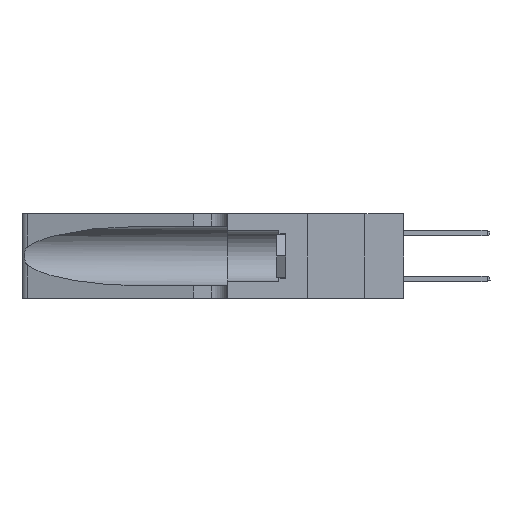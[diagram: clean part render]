
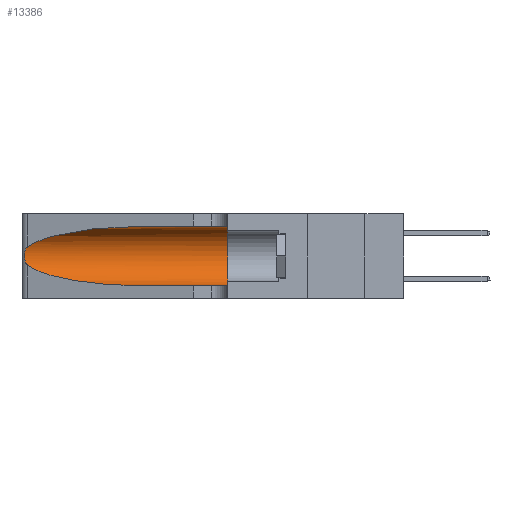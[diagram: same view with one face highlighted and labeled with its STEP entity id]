
A CAD part, left-side view. The second image highlights one B-rep face of the part: STEP entity #13386.
In plain terms, the highlighted cylindrical face has radius 3.308 mm (diameter 6.617 mm), a partial arc.
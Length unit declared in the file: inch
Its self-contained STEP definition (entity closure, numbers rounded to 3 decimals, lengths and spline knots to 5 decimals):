
#2082 = VERTEX_POINT ( 'NONE', #26902 ) ;
#2106 = EDGE_CURVE ( 'NONE', #43480, #2082, #8364, .T. ) ;
#2282 = AXIS2_PLACEMENT_3D ( 'NONE', #31212, #20043, #46346 ) ;
#2518 = CARTESIAN_POINT ( 'NONE',  ( 0.25639, 1.23184, 0.21858 ) ) ;
#4357 = CARTESIAN_POINT ( 'NONE',  ( 0.2373, 1.15595, 0.28018 ) ) ;
#4795 = DIRECTION ( 'NONE',  ( 0., -1., 0. ) ) ;
#5530 = CARTESIAN_POINT ( 'NONE',  ( 0.1305, 0.72297, 0.05475 ) ) ;
#5622 = VERTEX_POINT ( 'NONE', #33746 ) ;
#6374 = CARTESIAN_POINT ( 'NONE',  ( 0.25854, 1.2359, 0.20912 ) ) ;
#6934 = B_SPLINE_CURVE_WITH_KNOTS ( 'NONE', 3,
 ( #44008, #32668, #2518, #29024, #6374, #32831, #10190, #36622, #14015, #40368, #17830, #44166, #21634, #47950 ),
 .UNSPECIFIED., .F., .F.,
 ( 4, 2, 2, 2, 2, 2, 4 ),
 ( 0., 0.00027, 0.00053, 0.00107, 0.0016, 0.00187, 0.00214 ),
 .UNSPECIFIED. ) ;
#8364 = LINE ( 'NONE', #42034, #17282 ) ;
#10148 = CIRCLE ( 'NONE', #28569, 0.13025 ) ;
#10190 = CARTESIAN_POINT ( 'NONE',  ( 0.26075, 1.23896, 0.19203 ) ) ;
#13386 = ADVANCED_FACE ( 'NONE', ( #47611 ), #27585, .F. ) ;
#14015 = CARTESIAN_POINT ( 'NONE',  ( 0.26017, 1.23833, 0.17102 ) ) ;
#14213 = VECTOR ( 'NONE', #4795, 39.37008 ) ;
#15354 = CARTESIAN_POINT ( 'NONE',  ( 0.25487, 1.22718, 0.14631 ) ) ;
#15713 = CARTESIAN_POINT ( 'NONE',  ( 0.1305, 0.72297, 0.31525 ) ) ;
#15753 =( BOUNDED_CURVE ( )  B_SPLINE_CURVE ( 3, ( #20656, #20484, #28211, #5530 ),
 .UNSPECIFIED., .F., .F. ) 
 B_SPLINE_CURVE_WITH_KNOTS ( ( 4, 4 ),
 ( 3.44316, 4.71239 ),
 .UNSPECIFIED. ) 
 CURVE ( )  GEOMETRIC_REPRESENTATION_ITEM ( )  RATIONAL_B_SPLINE_CURVE ( ( 1., 0.87, 0.87, 1. ) ) 
 REPRESENTATION_ITEM ( '' )  );
#16607 = ORIENTED_EDGE ( 'NONE', *, *, #43605, .T. ) ;
#17282 = VECTOR ( 'NONE', #27069, 39.37008 ) ;
#17830 = CARTESIAN_POINT ( 'NONE',  ( 0.25789, 1.23486, 0.15765 ) ) ;
#19505 = CARTESIAN_POINT ( 'NONE',  ( 0.18966, 0.96281, 0.31525 ) ) ;
#19989 = CARTESIAN_POINT ( 'NONE',  ( 0.1305, 0.72297, 0.05475 ) ) ;
#20043 = DIRECTION ( 'NONE',  ( 0., -1., 0. ) ) ;
#20484 = CARTESIAN_POINT ( 'NONE',  ( 0.2373, 1.15595, 0.08982 ) ) ;
#20656 = CARTESIAN_POINT ( 'NONE',  ( 0.25487, 1.22718, 0.14631 ) ) ;
#20805 = DIRECTION ( 'NONE',  ( 0., 1., 0. ) ) ;
#21634 = CARTESIAN_POINT ( 'NONE',  ( 0.25555, 1.22993, 0.14849 ) ) ;
#24265 = CARTESIAN_POINT ( 'NONE',  ( 0.1305, 0.35, 0.31525 ) ) ;
#25650 = EDGE_CURVE ( 'NONE', #5622, #43592, #40740, .T. ) ;
#26902 = CARTESIAN_POINT ( 'NONE',  ( 0.1305, 0.35, 0.05475 ) ) ;
#27069 = DIRECTION ( 'NONE',  ( 0., -1., 0. ) ) ;
#27497 = CARTESIAN_POINT ( 'NONE',  ( 0.1305, 1.61858, 0.31525 ) ) ;
#27585 = CYLINDRICAL_SURFACE ( 'NONE', #2282, 0.13025 ) ;
#28211 = CARTESIAN_POINT ( 'NONE',  ( 0.18966, 0.96281, 0.05475 ) ) ;
#28569 = AXIS2_PLACEMENT_3D ( 'NONE', #43335, #20805, #47102 ) ;
#29024 = CARTESIAN_POINT ( 'NONE',  ( 0.25787, 1.23484, 0.2124 ) ) ;
#29061 = EDGE_CURVE ( 'NONE', #5622, #45926, #33306, .T. ) ;
#30831 = CARTESIAN_POINT ( 'NONE',  ( 0.25487, 1.22718, 0.22369 ) ) ;
#31212 = CARTESIAN_POINT ( 'NONE',  ( 0.1305, 1.61858, 0.185 ) ) ;
#32668 = CARTESIAN_POINT ( 'NONE',  ( 0.25555, 1.22994, 0.2215 ) ) ;
#32831 = CARTESIAN_POINT ( 'NONE',  ( 0.26018, 1.23835, 0.19895 ) ) ;
#33127 = ORIENTED_EDGE ( 'NONE', *, *, #29061, .T. ) ;
#33306 =( BOUNDED_CURVE ( )  B_SPLINE_CURVE ( 3, ( #15713, #19505, #4357, #30831 ),
 .UNSPECIFIED., .F., .T. ) 
 B_SPLINE_CURVE_WITH_KNOTS ( ( 4, 4 ),
 ( 1.5708, 2.84003 ),
 .UNSPECIFIED. ) 
 CURVE ( )  GEOMETRIC_REPRESENTATION_ITEM ( )  RATIONAL_B_SPLINE_CURVE ( ( 1., 0.87, 0.87, 1. ) ) 
 REPRESENTATION_ITEM ( '' )  );
#33746 = CARTESIAN_POINT ( 'NONE',  ( 0.1305, 0.72297, 0.31525 ) ) ;
#34301 = ORIENTED_EDGE ( 'NONE', *, *, #43754, .T. ) ;
#36622 = CARTESIAN_POINT ( 'NONE',  ( 0.26075, 1.23896, 0.178 ) ) ;
#39078 = EDGE_LOOP ( 'NONE', ( #33127, #34301, #16607, #46632, #47844, #40175 ) ) ;
#40175 = ORIENTED_EDGE ( 'NONE', *, *, #25650, .F. ) ;
#40368 = CARTESIAN_POINT ( 'NONE',  ( 0.25856, 1.23593, 0.16098 ) ) ;
#40740 = LINE ( 'NONE', #27497, #14213 ) ;
#41100 = EDGE_CURVE ( 'NONE', #43592, #2082, #10148, .T. ) ;
#42034 = CARTESIAN_POINT ( 'NONE',  ( 0.1305, 1.61858, 0.05475 ) ) ;
#43335 = CARTESIAN_POINT ( 'NONE',  ( 0.1305, 0.35, 0.185 ) ) ;
#43480 = VERTEX_POINT ( 'NONE', #19989 ) ;
#43592 = VERTEX_POINT ( 'NONE', #24265 ) ;
#43605 = EDGE_CURVE ( 'NONE', #45218, #43480, #15753, .T. ) ;
#43752 = CARTESIAN_POINT ( 'NONE',  ( 0.25487, 1.22718, 0.22369 ) ) ;
#43754 = EDGE_CURVE ( 'NONE', #45926, #45218, #6934, .T. ) ;
#44008 = CARTESIAN_POINT ( 'NONE',  ( 0.25487, 1.22718, 0.22369 ) ) ;
#44166 = CARTESIAN_POINT ( 'NONE',  ( 0.25639, 1.23186, 0.15144 ) ) ;
#45218 = VERTEX_POINT ( 'NONE', #15354 ) ;
#45926 = VERTEX_POINT ( 'NONE', #43752 ) ;
#46346 = DIRECTION ( 'NONE',  ( 0., 0., -1. ) ) ;
#46632 = ORIENTED_EDGE ( 'NONE', *, *, #2106, .T. ) ;
#47102 = DIRECTION ( 'NONE',  ( 0., 0., 1. ) ) ;
#47611 = FACE_OUTER_BOUND ( 'NONE', #39078, .T. ) ;
#47844 = ORIENTED_EDGE ( 'NONE', *, *, #41100, .F. ) ;
#47950 = CARTESIAN_POINT ( 'NONE',  ( 0.25487, 1.22718, 0.14631 ) ) ;
